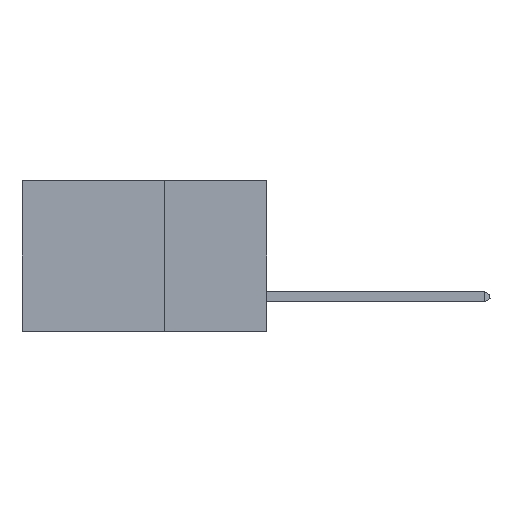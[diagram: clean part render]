
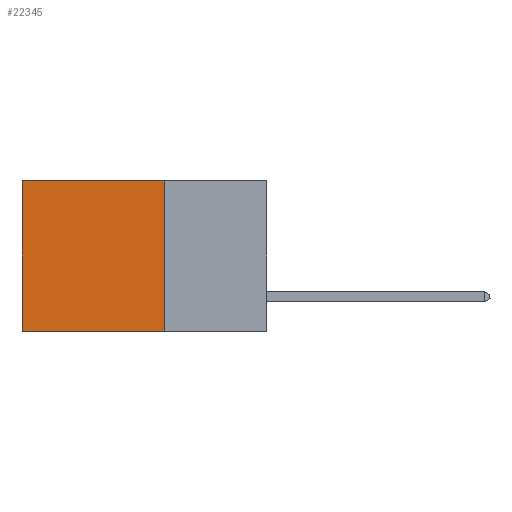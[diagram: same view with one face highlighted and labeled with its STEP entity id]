
A CAD part, left-side view. The second image highlights one B-rep face of the part: STEP entity #22345.
In plain terms, the highlighted planar face has unit normal (-1, 0, 0).
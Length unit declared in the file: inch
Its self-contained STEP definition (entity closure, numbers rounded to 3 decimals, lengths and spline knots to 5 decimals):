
#812 = EDGE_CURVE ( 'NONE', #9730, #16250, #9152, .T. ) ;
#1120 = CARTESIAN_POINT ( 'NONE',  ( 0.2875, 0.25, 0. ) ) ;
#1657 = PLANE ( 'NONE',  #3007 ) ;
#1910 = CARTESIAN_POINT ( 'NONE',  ( 0.2875, 0.25, 0. ) ) ;
#3007 = AXIS2_PLACEMENT_3D ( 'NONE', #1910, #18672, #7486 ) ;
#3520 = VERTEX_POINT ( 'NONE', #10932 ) ;
#3950 = ORIENTED_EDGE ( 'NONE', *, *, #15804, .F. ) ;
#5004 = EDGE_CURVE ( 'NONE', #3520, #16250, #9214, .T. ) ;
#6542 = LINE ( 'NONE', #9186, #14692 ) ;
#7094 = EDGE_LOOP ( 'NONE', ( #22581, #9897, #3950, #23250 ) ) ;
#7486 = DIRECTION ( 'NONE',  ( 0., 0., -1. ) ) ;
#7560 = DIRECTION ( 'NONE',  ( 0., 0., -1. ) ) ;
#8240 = CARTESIAN_POINT ( 'NONE',  ( 0.2875, 0.6, 0. ) ) ;
#9152 = LINE ( 'NONE', #8240, #12063 ) ;
#9186 = CARTESIAN_POINT ( 'NONE',  ( 0.2875, 0.25, 0. ) ) ;
#9214 = LINE ( 'NONE', #12877, #20353 ) ;
#9730 = VERTEX_POINT ( 'NONE', #22938 ) ;
#9897 = ORIENTED_EDGE ( 'NONE', *, *, #5004, .F. ) ;
#10932 = CARTESIAN_POINT ( 'NONE',  ( 0.2875, 0.25, -0.37 ) ) ;
#11710 = DIRECTION ( 'NONE',  ( 0., 0., -1. ) ) ;
#12063 = VECTOR ( 'NONE', #11710, 39.37008 ) ;
#12877 = CARTESIAN_POINT ( 'NONE',  ( 0.2875, 0.25, -0.37 ) ) ;
#14692 = VECTOR ( 'NONE', #7560, 39.37008 ) ;
#15804 = EDGE_CURVE ( 'NONE', #22164, #3520, #6542, .T. ) ;
#16106 = CARTESIAN_POINT ( 'NONE',  ( 0.2875, 0.6, -0.37 ) ) ;
#16140 = CARTESIAN_POINT ( 'NONE',  ( 0.2875, 0.25, 0. ) ) ;
#16250 = VERTEX_POINT ( 'NONE', #16106 ) ;
#16822 = LINE ( 'NONE', #1120, #17995 ) ;
#16914 = DIRECTION ( 'NONE',  ( 0., 1., 0. ) ) ;
#17977 = DIRECTION ( 'NONE',  ( 0., 1., 0. ) ) ;
#17995 = VECTOR ( 'NONE', #17977, 39.37008 ) ;
#18672 = DIRECTION ( 'NONE',  ( 1., 0., 0. ) ) ;
#20353 = VECTOR ( 'NONE', #16914, 39.37008 ) ;
#20444 = EDGE_CURVE ( 'NONE', #22164, #9730, #16822, .T. ) ;
#22164 = VERTEX_POINT ( 'NONE', #16140 ) ;
#22345 = ADVANCED_FACE ( 'NONE', ( #22723 ), #1657, .F. ) ;
#22581 = ORIENTED_EDGE ( 'NONE', *, *, #812, .T. ) ;
#22723 = FACE_OUTER_BOUND ( 'NONE', #7094, .T. ) ;
#22938 = CARTESIAN_POINT ( 'NONE',  ( 0.2875, 0.6, 0. ) ) ;
#23250 = ORIENTED_EDGE ( 'NONE', *, *, #20444, .T. ) ;
